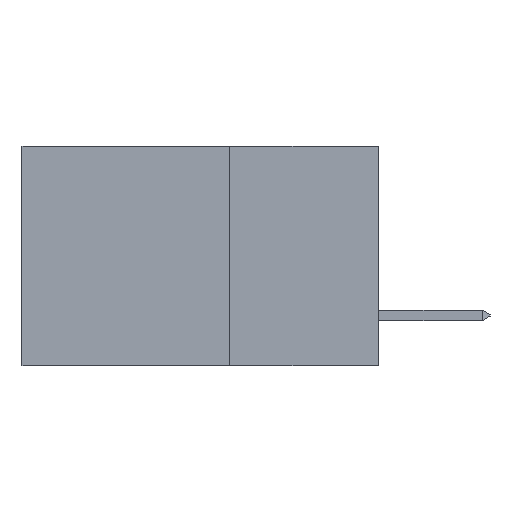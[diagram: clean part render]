
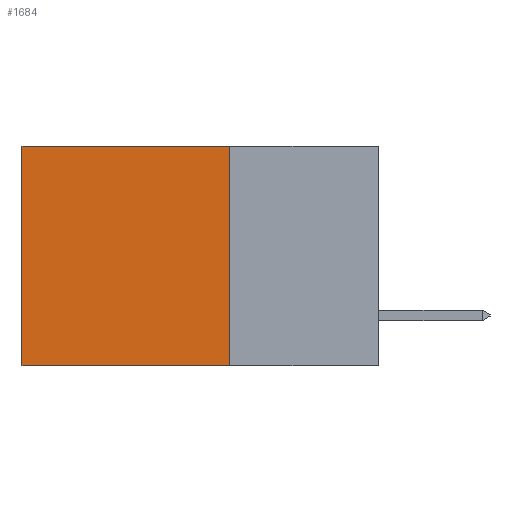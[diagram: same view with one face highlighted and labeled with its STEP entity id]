
A CAD part, left-side view. The second image highlights one B-rep face of the part: STEP entity #1684.
In plain terms, the highlighted planar face has unit normal (-1, 0, 0).
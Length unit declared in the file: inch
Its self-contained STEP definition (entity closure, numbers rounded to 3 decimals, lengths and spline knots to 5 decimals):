
#265 = VERTEX_POINT ( 'NONE', #9492 ) ;
#1489 = DIRECTION ( 'NONE',  ( 0., 1., 0. ) ) ;
#1684 = ADVANCED_FACE ( 'NONE', ( #12307 ), #9790, .F. ) ;
#1755 = AXIS2_PLACEMENT_3D ( 'NONE', #9681, #9666, #9651 ) ;
#2051 = CARTESIAN_POINT ( 'NONE',  ( 0.2615, 0.25, -0.37 ) ) ;
#2970 = VERTEX_POINT ( 'NONE', #9379 ) ;
#3194 = LINE ( 'NONE', #2051, #4833 ) ;
#3400 = CARTESIAN_POINT ( 'NONE',  ( 0.2615, 0.25, 0. ) ) ;
#3514 = LINE ( 'NONE', #3400, #5778 ) ;
#3979 = EDGE_CURVE ( 'NONE', #11542, #265, #3194, .T. ) ;
#4328 = DIRECTION ( 'NONE',  ( 0., 1., 0. ) ) ;
#4833 = VECTOR ( 'NONE', #1489, 39.37008 ) ;
#5762 = ORIENTED_EDGE ( 'NONE', *, *, #3979, .F. ) ;
#5778 = VECTOR ( 'NONE', #4328, 39.37008 ) ;
#6384 = EDGE_CURVE ( 'NONE', #2970, #11542, #9598, .T. ) ;
#6490 = VERTEX_POINT ( 'NONE', #10179 ) ;
#6792 = VECTOR ( 'NONE', #8123, 39.37008 ) ;
#6828 = ORIENTED_EDGE ( 'NONE', *, *, #11640, .T. ) ;
#6981 = LINE ( 'NONE', #12177, #11679 ) ;
#7529 = ORIENTED_EDGE ( 'NONE', *, *, #9843, .T. ) ;
#8123 = DIRECTION ( 'NONE',  ( 0., 0., -1. ) ) ;
#8451 = DIRECTION ( 'NONE',  ( 0., 0., -1. ) ) ;
#9379 = CARTESIAN_POINT ( 'NONE',  ( 0.2615, 0.25, 0. ) ) ;
#9492 = CARTESIAN_POINT ( 'NONE',  ( 0.2615, 0.6, -0.37 ) ) ;
#9598 = LINE ( 'NONE', #11883, #6792 ) ;
#9651 = DIRECTION ( 'NONE',  ( 0., 0., -1. ) ) ;
#9666 = DIRECTION ( 'NONE',  ( 1., 0., 0. ) ) ;
#9681 = CARTESIAN_POINT ( 'NONE',  ( 0.2615, 0.25, -0.37 ) ) ;
#9790 = PLANE ( 'NONE',  #1755 ) ;
#9843 = EDGE_CURVE ( 'NONE', #6490, #265, #6981, .T. ) ;
#10179 = CARTESIAN_POINT ( 'NONE',  ( 0.2615, 0.6, 0. ) ) ;
#10870 = CARTESIAN_POINT ( 'NONE',  ( 0.2615, 0.25, -0.37 ) ) ;
#11542 = VERTEX_POINT ( 'NONE', #10870 ) ;
#11640 = EDGE_CURVE ( 'NONE', #2970, #6490, #3514, .T. ) ;
#11679 = VECTOR ( 'NONE', #8451, 39.37008 ) ;
#11883 = CARTESIAN_POINT ( 'NONE',  ( 0.2615, 0.25, -0.37 ) ) ;
#12046 = ORIENTED_EDGE ( 'NONE', *, *, #6384, .F. ) ;
#12177 = CARTESIAN_POINT ( 'NONE',  ( 0.2615, 0.6, -0.37 ) ) ;
#12307 = FACE_OUTER_BOUND ( 'NONE', #12442, .T. ) ;
#12442 = EDGE_LOOP ( 'NONE', ( #7529, #5762, #12046, #6828 ) ) ;
